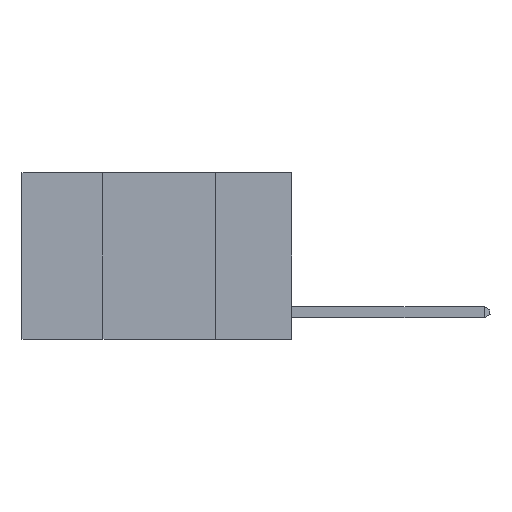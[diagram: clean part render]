
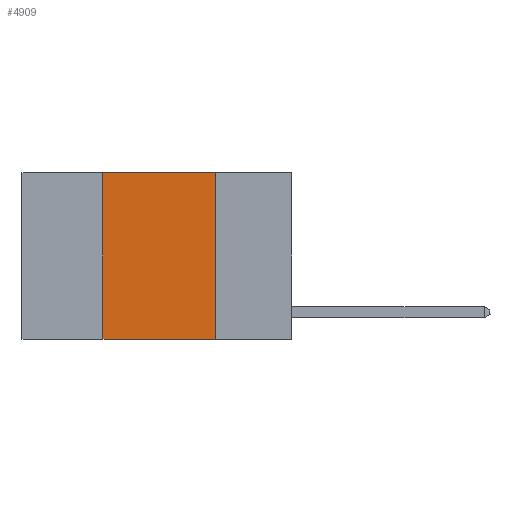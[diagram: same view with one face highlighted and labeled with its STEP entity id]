
A CAD part, left-side view. The second image highlights one B-rep face of the part: STEP entity #4909.
In plain terms, the highlighted planar face has unit normal (-1, 0, 0).
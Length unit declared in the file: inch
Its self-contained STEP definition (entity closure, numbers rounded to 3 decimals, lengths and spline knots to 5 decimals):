
#210 = VERTEX_POINT ( 'NONE', #3905 ) ;
#632 = AXIS2_PLACEMENT_3D ( 'NONE', #8910, #3363, #6154 ) ;
#661 = VECTOR ( 'NONE', #1115, 39.37008 ) ;
#806 = DIRECTION ( 'NONE',  ( 0., -1., 0. ) ) ;
#924 = EDGE_CURVE ( 'NONE', #210, #1026, #3427, .T. ) ;
#1026 = VERTEX_POINT ( 'NONE', #1647 ) ;
#1112 = EDGE_CURVE ( 'NONE', #1026, #5687, #8920, .T. ) ;
#1115 = DIRECTION ( 'NONE',  ( 0., 0., 1. ) ) ;
#1285 = CARTESIAN_POINT ( 'NONE',  ( 0., 0.42, 0. ) ) ;
#1292 = ORIENTED_EDGE ( 'NONE', *, *, #7500, .F. ) ;
#1647 = CARTESIAN_POINT ( 'NONE',  ( 0., 0.17, 0. ) ) ;
#1927 = DIRECTION ( 'NONE',  ( 0., 0., -1. ) ) ;
#2075 = CARTESIAN_POINT ( 'NONE',  ( 0., 0.6, -0.37 ) ) ;
#2165 = VERTEX_POINT ( 'NONE', #4998 ) ;
#2337 = EDGE_LOOP ( 'NONE', ( #3045, #4055, #1292, #4421 ) ) ;
#2755 = DIRECTION ( 'NONE',  ( 0., -1., 0. ) ) ;
#2855 = LINE ( 'NONE', #2075, #3132 ) ;
#3045 = ORIENTED_EDGE ( 'NONE', *, *, #1112, .F. ) ;
#3132 = VECTOR ( 'NONE', #806, 39.37008 ) ;
#3259 = CARTESIAN_POINT ( 'NONE',  ( 0., 0.17, -0.37 ) ) ;
#3284 = PLANE ( 'NONE',  #632 ) ;
#3363 = DIRECTION ( 'NONE',  ( 1., 0., 0. ) ) ;
#3427 = LINE ( 'NONE', #9115, #5410 ) ;
#3898 = VECTOR ( 'NONE', #1927, 39.37008 ) ;
#3905 = CARTESIAN_POINT ( 'NONE',  ( 0., 0.42, 0. ) ) ;
#3920 = LINE ( 'NONE', #1285, #661 ) ;
#4055 = ORIENTED_EDGE ( 'NONE', *, *, #924, .F. ) ;
#4421 = ORIENTED_EDGE ( 'NONE', *, *, #7252, .T. ) ;
#4909 = ADVANCED_FACE ( 'NONE', ( #7596 ), #3284, .F. ) ;
#4998 = CARTESIAN_POINT ( 'NONE',  ( 0., 0.42, -0.37 ) ) ;
#5410 = VECTOR ( 'NONE', #2755, 39.37008 ) ;
#5687 = VERTEX_POINT ( 'NONE', #3259 ) ;
#6154 = DIRECTION ( 'NONE',  ( 0., 0., -1. ) ) ;
#7252 = EDGE_CURVE ( 'NONE', #2165, #5687, #2855, .T. ) ;
#7500 = EDGE_CURVE ( 'NONE', #2165, #210, #3920, .T. ) ;
#7596 = FACE_OUTER_BOUND ( 'NONE', #2337, .T. ) ;
#8827 = CARTESIAN_POINT ( 'NONE',  ( 0., 0.17, 0. ) ) ;
#8910 = CARTESIAN_POINT ( 'NONE',  ( 0., 0.6, 0. ) ) ;
#8920 = LINE ( 'NONE', #8827, #3898 ) ;
#9115 = CARTESIAN_POINT ( 'NONE',  ( 0., 0.6, 0. ) ) ;
